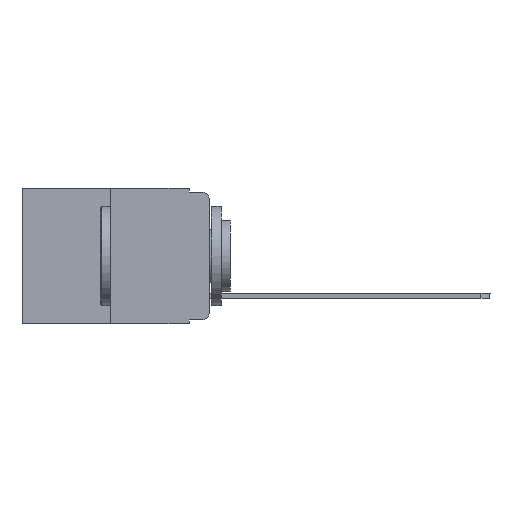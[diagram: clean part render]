
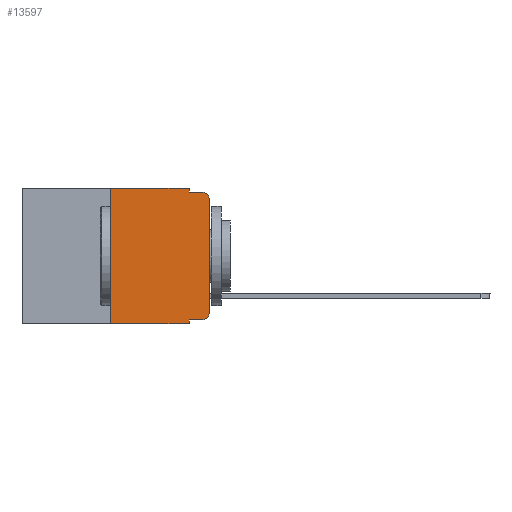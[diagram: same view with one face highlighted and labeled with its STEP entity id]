
A CAD part, left-side view. The second image highlights one B-rep face of the part: STEP entity #13597.
In plain terms, the highlighted planar face has unit normal (-1, 0, 0).
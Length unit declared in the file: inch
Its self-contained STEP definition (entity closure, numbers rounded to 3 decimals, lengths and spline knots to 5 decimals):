
#74 = DIRECTION ( 'NONE',  ( 0., 0., 1. ) ) ;
#185 = CIRCLE ( 'NONE', #3020, 0.02 ) ;
#209 = CARTESIAN_POINT ( 'NONE',  ( 0., 0.02, -0.333 ) ) ;
#472 = LINE ( 'NONE', #11553, #15792 ) ;
#528 = VERTEX_POINT ( 'NONE', #7051 ) ;
#867 = DIRECTION ( 'NONE',  ( 1., 0., 0. ) ) ;
#1005 = CARTESIAN_POINT ( 'NONE',  ( 0., 0.051, -0.01 ) ) ;
#1029 = DIRECTION ( 'NONE',  ( 0., -1., 0. ) ) ;
#1084 = CARTESIAN_POINT ( 'NONE',  ( 0., 0.473, -0.343 ) ) ;
#1840 = DIRECTION ( 'NONE',  ( 0., 0., -1. ) ) ;
#1961 = CARTESIAN_POINT ( 'NONE',  ( 0., 0.051, -0.343 ) ) ;
#1984 = DIRECTION ( 'NONE',  ( 0., -1., 0. ) ) ;
#3020 = AXIS2_PLACEMENT_3D ( 'NONE', #13312, #5690, #14596 ) ;
#3169 = EDGE_CURVE ( 'NONE', #4301, #11904, #15327, .T. ) ;
#3381 = CARTESIAN_POINT ( 'NONE',  ( 0., 0.02, -0.313 ) ) ;
#3519 = DIRECTION ( 'NONE',  ( 0., 0., -1. ) ) ;
#3533 = CARTESIAN_POINT ( 'NONE',  ( 0., 0.051, -0.01 ) ) ;
#4014 = VECTOR ( 'NONE', #74, 39.37008 ) ;
#4015 = CARTESIAN_POINT ( 'NONE',  ( 0., 0.25, 0. ) ) ;
#4144 = EDGE_LOOP ( 'NONE', ( #14908, #6612, #12000, #11029, #5324, #13300, #11342, #15595, #14778, #13158 ) ) ;
#4301 = VERTEX_POINT ( 'NONE', #209 ) ;
#4480 = VERTEX_POINT ( 'NONE', #7852 ) ;
#4958 = LINE ( 'NONE', #11635, #7746 ) ;
#5083 = VERTEX_POINT ( 'NONE', #1961 ) ;
#5315 = VECTOR ( 'NONE', #5550, 39.37008 ) ;
#5324 = ORIENTED_EDGE ( 'NONE', *, *, #6968, .F. ) ;
#5360 = VECTOR ( 'NONE', #12447, 39.37008 ) ;
#5550 = DIRECTION ( 'NONE',  ( 0., 0., 1. ) ) ;
#5690 = DIRECTION ( 'NONE',  ( -1., 0., 0. ) ) ;
#5925 = DIRECTION ( 'NONE',  ( 0., 0., -1. ) ) ;
#6227 = LINE ( 'NONE', #4015, #4014 ) ;
#6274 = VECTOR ( 'NONE', #1029, 39.37008 ) ;
#6612 = ORIENTED_EDGE ( 'NONE', *, *, #15193, .T. ) ;
#6672 = EDGE_CURVE ( 'NONE', #528, #5083, #11020, .T. ) ;
#6709 = LINE ( 'NONE', #13291, #5315 ) ;
#6968 = EDGE_CURVE ( 'NONE', #4480, #7330, #472, .T. ) ;
#7051 = CARTESIAN_POINT ( 'NONE',  ( 0., 0.25, -0.343 ) ) ;
#7092 = CARTESIAN_POINT ( 'NONE',  ( 0., 0.051, 0. ) ) ;
#7170 = AXIS2_PLACEMENT_3D ( 'NONE', #3381, #13381, #12221 ) ;
#7330 = VERTEX_POINT ( 'NONE', #11793 ) ;
#7746 = VECTOR ( 'NONE', #1840, 39.37008 ) ;
#7852 = CARTESIAN_POINT ( 'NONE',  ( 0., 0.25, 0. ) ) ;
#8015 = AXIS2_PLACEMENT_3D ( 'NONE', #12255, #867, #3519 ) ;
#8232 = VERTEX_POINT ( 'NONE', #9193 ) ;
#8267 = EDGE_CURVE ( 'NONE', #528, #4480, #6227, .T. ) ;
#8347 = VECTOR ( 'NONE', #5925, 39.37008 ) ;
#8353 = LINE ( 'NONE', #3533, #5360 ) ;
#8511 = CARTESIAN_POINT ( 'NONE',  ( 0., 0.02, -0.01 ) ) ;
#8948 = LINE ( 'NONE', #7092, #8347 ) ;
#9193 = CARTESIAN_POINT ( 'NONE',  ( 0., 0., -0.03 ) ) ;
#9237 = EDGE_CURVE ( 'NONE', #10788, #4301, #15320, .T. ) ;
#9439 = EDGE_CURVE ( 'NONE', #10763, #10800, #8353, .T. ) ;
#10484 = EDGE_CURVE ( 'NONE', #11904, #8232, #6709, .T. ) ;
#10763 = VERTEX_POINT ( 'NONE', #1005 ) ;
#10788 = VERTEX_POINT ( 'NONE', #11278 ) ;
#10800 = VERTEX_POINT ( 'NONE', #8511 ) ;
#11020 = LINE ( 'NONE', #1084, #6274 ) ;
#11029 = ORIENTED_EDGE ( 'NONE', *, *, #15215, .F. ) ;
#11278 = CARTESIAN_POINT ( 'NONE',  ( 0., 0.051, -0.333 ) ) ;
#11342 = ORIENTED_EDGE ( 'NONE', *, *, #6672, .T. ) ;
#11438 = DIRECTION ( 'NONE',  ( 0., -1., 0. ) ) ;
#11553 = CARTESIAN_POINT ( 'NONE',  ( 0., 0.473, 0. ) ) ;
#11635 = CARTESIAN_POINT ( 'NONE',  ( 0., 0.051, 0. ) ) ;
#11793 = CARTESIAN_POINT ( 'NONE',  ( 0., 0.051, 0. ) ) ;
#11904 = VERTEX_POINT ( 'NONE', #15803 ) ;
#12000 = ORIENTED_EDGE ( 'NONE', *, *, #9439, .F. ) ;
#12221 = DIRECTION ( 'NONE',  ( 0., 0., -1. ) ) ;
#12255 = CARTESIAN_POINT ( 'NONE',  ( 0., 0.473, 0. ) ) ;
#12447 = DIRECTION ( 'NONE',  ( 0., -1., 0. ) ) ;
#13158 = ORIENTED_EDGE ( 'NONE', *, *, #3169, .T. ) ;
#13291 = CARTESIAN_POINT ( 'NONE',  ( 0., 0., 0. ) ) ;
#13300 = ORIENTED_EDGE ( 'NONE', *, *, #8267, .F. ) ;
#13312 = CARTESIAN_POINT ( 'NONE',  ( 0., 0.02, -0.03 ) ) ;
#13381 = DIRECTION ( 'NONE',  ( -1., 0., 0. ) ) ;
#13597 = ADVANCED_FACE ( 'NONE', ( #15756 ), #14817, .F. ) ;
#14528 = VECTOR ( 'NONE', #1984, 39.37008 ) ;
#14596 = DIRECTION ( 'NONE',  ( 0., 0., -1. ) ) ;
#14778 = ORIENTED_EDGE ( 'NONE', *, *, #9237, .T. ) ;
#14817 = PLANE ( 'NONE',  #8015 ) ;
#14908 = ORIENTED_EDGE ( 'NONE', *, *, #10484, .T. ) ;
#15193 = EDGE_CURVE ( 'NONE', #8232, #10800, #185, .T. ) ;
#15215 = EDGE_CURVE ( 'NONE', #7330, #10763, #8948, .T. ) ;
#15320 = LINE ( 'NONE', #15874, #14528 ) ;
#15327 = CIRCLE ( 'NONE', #7170, 0.02 ) ;
#15595 = ORIENTED_EDGE ( 'NONE', *, *, #15739, .F. ) ;
#15739 = EDGE_CURVE ( 'NONE', #10788, #5083, #4958, .T. ) ;
#15756 = FACE_OUTER_BOUND ( 'NONE', #4144, .T. ) ;
#15792 = VECTOR ( 'NONE', #11438, 39.37008 ) ;
#15803 = CARTESIAN_POINT ( 'NONE',  ( 0., 0., -0.313 ) ) ;
#15874 = CARTESIAN_POINT ( 'NONE',  ( 0., 0.051, -0.333 ) ) ;
